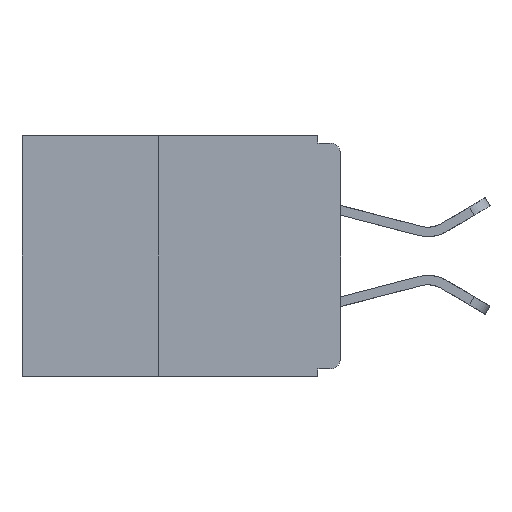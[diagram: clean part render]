
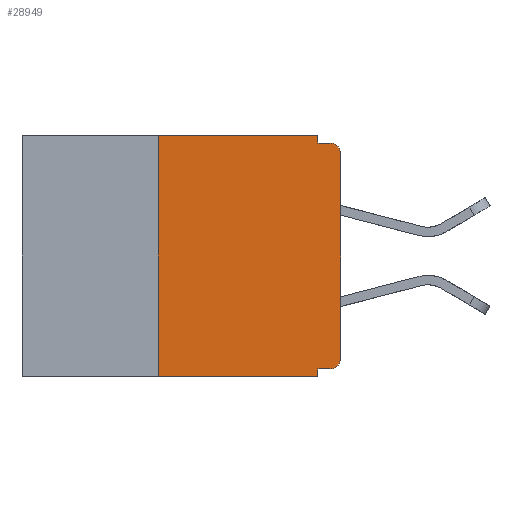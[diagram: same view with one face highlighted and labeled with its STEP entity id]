
A CAD part, left-side view. The second image highlights one B-rep face of the part: STEP entity #28949.
In plain terms, the highlighted planar face has unit normal (-1, 0, 0).
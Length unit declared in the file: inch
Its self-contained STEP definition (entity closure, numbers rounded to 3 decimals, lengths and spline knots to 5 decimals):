
#305 = CARTESIAN_POINT ( 'NONE',  ( 0., 0.031, 0. ) ) ;
#442 = CARTESIAN_POINT ( 'NONE',  ( 0., 0.031, -0.33 ) ) ;
#464 = EDGE_CURVE ( 'NONE', #2286, #25871, #1136, .T. ) ;
#750 = DIRECTION ( 'NONE',  ( 0., 0., -1. ) ) ;
#1113 = DIRECTION ( 'NONE',  ( 0., -1., 0. ) ) ;
#1136 = LINE ( 'NONE', #13073, #13490 ) ;
#1388 = EDGE_CURVE ( 'NONE', #20686, #2129, #25853, .T. ) ;
#1692 = DIRECTION ( 'NONE',  ( 0., -1., 0. ) ) ;
#2076 = CARTESIAN_POINT ( 'NONE',  ( 0., 0., -0.32 ) ) ;
#2129 = VERTEX_POINT ( 'NONE', #5925 ) ;
#2286 = VERTEX_POINT ( 'NONE', #31149 ) ;
#2970 = ORIENTED_EDGE ( 'NONE', *, *, #26841, .F. ) ;
#3114 = CARTESIAN_POINT ( 'NONE',  ( 0., 0.25, -0.33 ) ) ;
#3510 = CARTESIAN_POINT ( 'NONE',  ( 0., 0., 0. ) ) ;
#4623 = ORIENTED_EDGE ( 'NONE', *, *, #464, .F. ) ;
#4973 = ORIENTED_EDGE ( 'NONE', *, *, #19028, .T. ) ;
#5075 = EDGE_CURVE ( 'NONE', #2129, #21115, #13103, .T. ) ;
#5260 = CARTESIAN_POINT ( 'NONE',  ( 0., 0.015, -0.305 ) ) ;
#5483 = VERTEX_POINT ( 'NONE', #15491 ) ;
#5591 = CARTESIAN_POINT ( 'NONE',  ( 0., 0.031, 0. ) ) ;
#5649 = PLANE ( 'NONE',  #25700 ) ;
#5717 = ORIENTED_EDGE ( 'NONE', *, *, #20324, .T. ) ;
#5871 = VECTOR ( 'NONE', #30716, 39.37008 ) ;
#5925 = CARTESIAN_POINT ( 'NONE',  ( 0., 0.031, -0.01 ) ) ;
#6599 = ORIENTED_EDGE ( 'NONE', *, *, #16876, .F. ) ;
#6636 = LINE ( 'NONE', #3510, #5871 ) ;
#6954 = CARTESIAN_POINT ( 'NONE',  ( 0., 0.015, -0.01 ) ) ;
#7210 = CIRCLE ( 'NONE', #11971, 0.015 ) ;
#7594 = VERTEX_POINT ( 'NONE', #19240 ) ;
#7724 = DIRECTION ( 'NONE',  ( 0., 0., -1. ) ) ;
#9929 = VECTOR ( 'NONE', #12983, 39.37008 ) ;
#10335 = CARTESIAN_POINT ( 'NONE',  ( 0., 0.25, 0. ) ) ;
#10371 = EDGE_LOOP ( 'NONE', ( #4973, #12589, #21407, #20559, #6599, #25331, #5717, #4623, #2970, #19080 ) ) ;
#10831 = VERTEX_POINT ( 'NONE', #11973 ) ;
#11971 = AXIS2_PLACEMENT_3D ( 'NONE', #5260, #22556, #7724 ) ;
#11973 = CARTESIAN_POINT ( 'NONE',  ( 0., 0.25, -0.33 ) ) ;
#12589 = ORIENTED_EDGE ( 'NONE', *, *, #29223, .T. ) ;
#12983 = DIRECTION ( 'NONE',  ( 0., 0., 1. ) ) ;
#13073 = CARTESIAN_POINT ( 'NONE',  ( 0., 0.031, -0.33 ) ) ;
#13103 = LINE ( 'NONE', #22593, #25542 ) ;
#13490 = VECTOR ( 'NONE', #29451, 39.37008 ) ;
#14225 = CARTESIAN_POINT ( 'NONE',  ( 0., 0.015, -0.025 ) ) ;
#14258 = VERTEX_POINT ( 'NONE', #10335 ) ;
#14826 = LINE ( 'NONE', #18427, #28002 ) ;
#14852 = CIRCLE ( 'NONE', #23415, 0.015 ) ;
#15491 = CARTESIAN_POINT ( 'NONE',  ( 0., 0.015, -0.32 ) ) ;
#15567 = DIRECTION ( 'NONE',  ( 1., 0., 0. ) ) ;
#16503 = CARTESIAN_POINT ( 'NONE',  ( 0., 0.437, -0.33 ) ) ;
#16516 = LINE ( 'NONE', #3114, #9929 ) ;
#16734 = DIRECTION ( 'NONE',  ( 0., 0., -1. ) ) ;
#16876 = EDGE_CURVE ( 'NONE', #14258, #20686, #14826, .T. ) ;
#17711 = VECTOR ( 'NONE', #26502, 39.37008 ) ;
#18427 = CARTESIAN_POINT ( 'NONE',  ( 0., 0.437, 0. ) ) ;
#18925 = VECTOR ( 'NONE', #1692, 39.37008 ) ;
#19028 = EDGE_CURVE ( 'NONE', #19966, #7594, #6636, .T. ) ;
#19080 = ORIENTED_EDGE ( 'NONE', *, *, #28150, .T. ) ;
#19240 = CARTESIAN_POINT ( 'NONE',  ( 0., 0., -0.025 ) ) ;
#19966 = VERTEX_POINT ( 'NONE', #19982 ) ;
#19982 = CARTESIAN_POINT ( 'NONE',  ( 0., 0., -0.305 ) ) ;
#20277 = VECTOR ( 'NONE', #26718, 39.37008 ) ;
#20324 = EDGE_CURVE ( 'NONE', #10831, #25871, #25510, .T. ) ;
#20559 = ORIENTED_EDGE ( 'NONE', *, *, #1388, .F. ) ;
#20686 = VERTEX_POINT ( 'NONE', #5591 ) ;
#21115 = VERTEX_POINT ( 'NONE', #6954 ) ;
#21407 = ORIENTED_EDGE ( 'NONE', *, *, #5075, .F. ) ;
#22556 = DIRECTION ( 'NONE',  ( -1., 0., 0. ) ) ;
#22593 = CARTESIAN_POINT ( 'NONE',  ( 0., 0., -0.01 ) ) ;
#22610 = DIRECTION ( 'NONE',  ( 0., -1., 0. ) ) ;
#22636 = FACE_OUTER_BOUND ( 'NONE', #10371, .T. ) ;
#23415 = AXIS2_PLACEMENT_3D ( 'NONE', #14225, #31534, #16734 ) ;
#25273 = EDGE_CURVE ( 'NONE', #10831, #14258, #16516, .T. ) ;
#25331 = ORIENTED_EDGE ( 'NONE', *, *, #25273, .F. ) ;
#25510 = LINE ( 'NONE', #16503, #18925 ) ;
#25542 = VECTOR ( 'NONE', #22610, 39.37008 ) ;
#25700 = AXIS2_PLACEMENT_3D ( 'NONE', #30381, #15567, #750 ) ;
#25853 = LINE ( 'NONE', #305, #17711 ) ;
#25871 = VERTEX_POINT ( 'NONE', #442 ) ;
#26502 = DIRECTION ( 'NONE',  ( 0., 0., -1. ) ) ;
#26718 = DIRECTION ( 'NONE',  ( 0., 1., 0. ) ) ;
#26841 = EDGE_CURVE ( 'NONE', #5483, #2286, #27625, .T. ) ;
#27625 = LINE ( 'NONE', #2076, #20277 ) ;
#28002 = VECTOR ( 'NONE', #1113, 39.37008 ) ;
#28150 = EDGE_CURVE ( 'NONE', #5483, #19966, #7210, .T. ) ;
#28949 = ADVANCED_FACE ( 'NONE', ( #22636 ), #5649, .F. ) ;
#29223 = EDGE_CURVE ( 'NONE', #7594, #21115, #14852, .T. ) ;
#29451 = DIRECTION ( 'NONE',  ( 0., 0., -1. ) ) ;
#30381 = CARTESIAN_POINT ( 'NONE',  ( 0., 0.437, 0. ) ) ;
#30716 = DIRECTION ( 'NONE',  ( 0., 0., 1. ) ) ;
#31149 = CARTESIAN_POINT ( 'NONE',  ( 0., 0.031, -0.32 ) ) ;
#31534 = DIRECTION ( 'NONE',  ( -1., 0., 0. ) ) ;
